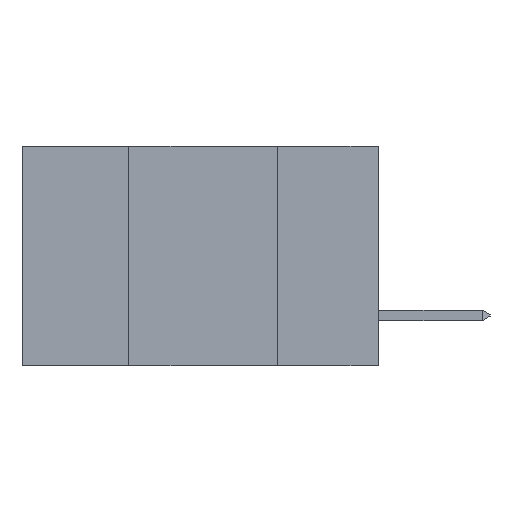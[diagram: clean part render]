
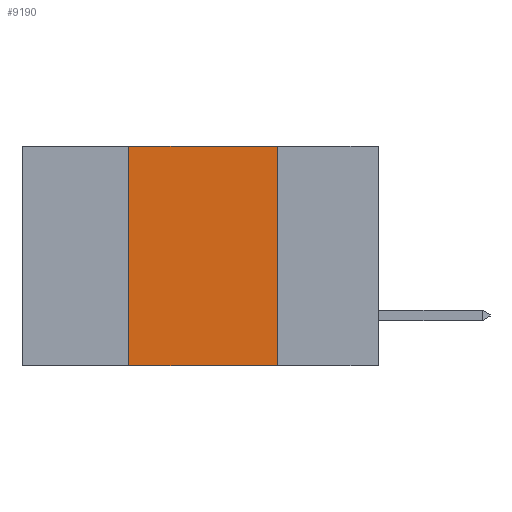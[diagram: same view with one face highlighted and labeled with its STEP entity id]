
A CAD part, left-side view. The second image highlights one B-rep face of the part: STEP entity #9190.
In plain terms, the highlighted planar face has unit normal (-1, 0, 0).
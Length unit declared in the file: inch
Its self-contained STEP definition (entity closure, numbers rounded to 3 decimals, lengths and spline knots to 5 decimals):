
#376 = VERTEX_POINT ( 'NONE', #6746 ) ;
#1596 = EDGE_CURVE ( 'NONE', #376, #4332, #4669, .T. ) ;
#1843 = CARTESIAN_POINT ( 'NONE',  ( 0., 0.17, 0. ) ) ;
#1958 = EDGE_CURVE ( 'NONE', #8211, #5511, #5204, .T. ) ;
#1973 = CARTESIAN_POINT ( 'NONE',  ( 0., 0.42, 0. ) ) ;
#2143 = CARTESIAN_POINT ( 'NONE',  ( 0., 0.42, -0.37 ) ) ;
#2617 = CARTESIAN_POINT ( 'NONE',  ( 0., 0.6, 0. ) ) ;
#2786 = LINE ( 'NONE', #1843, #11829 ) ;
#3169 = ORIENTED_EDGE ( 'NONE', *, *, #1958, .T. ) ;
#3286 = LINE ( 'NONE', #1973, #7725 ) ;
#3600 = DIRECTION ( 'NONE',  ( 0., 0., -1. ) ) ;
#3815 = ORIENTED_EDGE ( 'NONE', *, *, #6371, .F. ) ;
#3852 = ORIENTED_EDGE ( 'NONE', *, *, #8046, .F. ) ;
#4332 = VERTEX_POINT ( 'NONE', #10714 ) ;
#4555 = FACE_OUTER_BOUND ( 'NONE', #6913, .T. ) ;
#4669 = LINE ( 'NONE', #6410, #8943 ) ;
#4774 = DIRECTION ( 'NONE',  ( 0., 0., -1. ) ) ;
#5204 = LINE ( 'NONE', #6970, #7763 ) ;
#5237 = ORIENTED_EDGE ( 'NONE', *, *, #1596, .F. ) ;
#5511 = VERTEX_POINT ( 'NONE', #6930 ) ;
#5608 = DIRECTION ( 'NONE',  ( 0., -1., 0. ) ) ;
#6243 = AXIS2_PLACEMENT_3D ( 'NONE', #2617, #8827, #3600 ) ;
#6371 = EDGE_CURVE ( 'NONE', #8211, #376, #3286, .T. ) ;
#6410 = CARTESIAN_POINT ( 'NONE',  ( 0., 0.6, 0. ) ) ;
#6746 = CARTESIAN_POINT ( 'NONE',  ( 0., 0.42, 0. ) ) ;
#6913 = EDGE_LOOP ( 'NONE', ( #3852, #5237, #3815, #3169 ) ) ;
#6930 = CARTESIAN_POINT ( 'NONE',  ( 0., 0.17, -0.37 ) ) ;
#6970 = CARTESIAN_POINT ( 'NONE',  ( 0., 0.6, -0.37 ) ) ;
#7725 = VECTOR ( 'NONE', #9533, 39.37008 ) ;
#7763 = VECTOR ( 'NONE', #10458, 39.37008 ) ;
#8046 = EDGE_CURVE ( 'NONE', #4332, #5511, #2786, .T. ) ;
#8211 = VERTEX_POINT ( 'NONE', #2143 ) ;
#8827 = DIRECTION ( 'NONE',  ( 1., 0., 0. ) ) ;
#8943 = VECTOR ( 'NONE', #5608, 39.37008 ) ;
#9190 = ADVANCED_FACE ( 'NONE', ( #4555 ), #11373, .F. ) ;
#9533 = DIRECTION ( 'NONE',  ( 0., 0., 1. ) ) ;
#10458 = DIRECTION ( 'NONE',  ( 0., -1., 0. ) ) ;
#10714 = CARTESIAN_POINT ( 'NONE',  ( 0., 0.17, 0. ) ) ;
#11373 = PLANE ( 'NONE',  #6243 ) ;
#11829 = VECTOR ( 'NONE', #4774, 39.37008 ) ;
